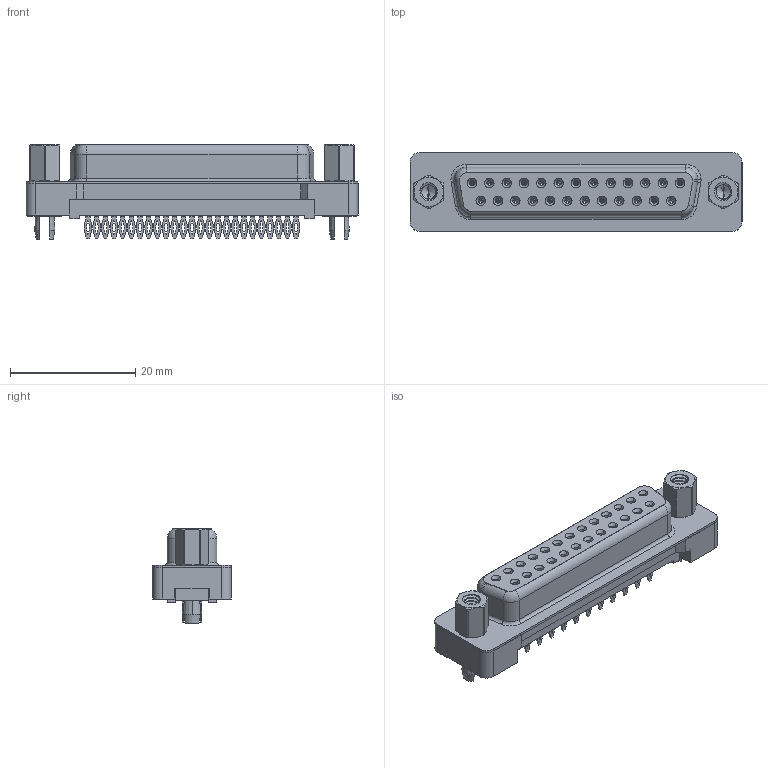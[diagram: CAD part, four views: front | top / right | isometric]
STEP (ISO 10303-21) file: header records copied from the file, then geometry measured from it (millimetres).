
FILE_DESCRIPTION (( 'STEP AP203' ), '1' );
FILE_NAME ('628-025-326-017.STEP', '2020-07-16T00:04:37', ( '' ), ( '' ), 'SwSTEP 2.0', 'SolidWorks 2020', '' );
FILE_SCHEMA (( 'CONFIG_CONTROL_DESIGN' ));
Length unit declared in the file: millimetre
Products named in the file (7): 628 4-40 Hex Standoff; 628 PB Contact Row 1_26; 628 PB Contact Row 2_26; 628 PB 4-40 Threaded Rivet with Boardlock; 628 PB Shell_25 Contacts; 628-025-326-017; 628 Plastic Body Housing_25 Contacts
Assembly tree (31 placements, depth 2):
  628-025-326-017
    628 Plastic Body Housing_25 Contacts
    628 PB Shell_25 Contacts
    628 PB Contact Row 1_26  x13
    628 PB Contact Row 2_26  x12
    628 4-40 Hex Standoff  x2
    628 PB 4-40 Threaded Rivet with Boardlock  x2
Bounding box: 53.05 x 12.55 x 15.05 mm (x, y, z)
Volume: 3529.7 mm3; surface area: 9045.4 mm2
Topology: 31 solids, 31 shells, 2637 faces, 6475 edges, 3938 vertices
Faces by surface type: plane 1056, cylinder 670, bspline 568, torus 176, cone 167
Entity records: 25982 total; most frequent: CARTESIAN_POINT 9010, ORIENTED_EDGE 3304, DIRECTION 3106, EDGE_CURVE 1652, AXIS2_PLACEMENT_3D 1076, VERTEX_POINT 1038, VECTOR 954, LINE 954
